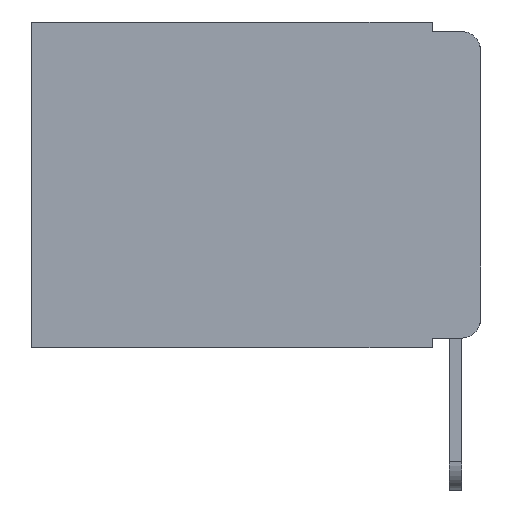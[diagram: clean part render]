
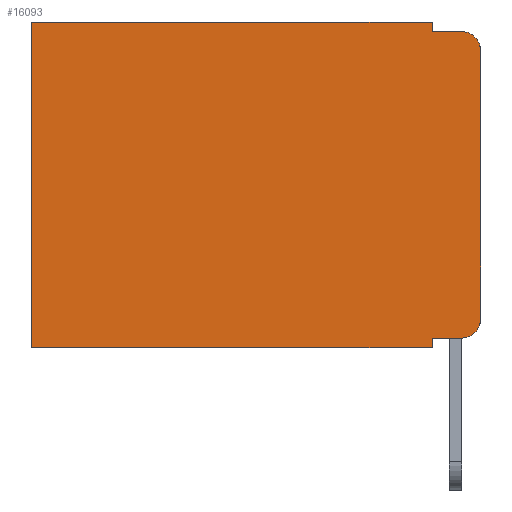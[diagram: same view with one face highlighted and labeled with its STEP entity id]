
A CAD part, left-side view. The second image highlights one B-rep face of the part: STEP entity #16093.
In plain terms, the highlighted planar face has unit normal (-1, 0, 0).
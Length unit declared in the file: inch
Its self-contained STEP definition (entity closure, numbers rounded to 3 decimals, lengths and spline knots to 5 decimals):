
#218 = DIRECTION ( 'NONE',  ( 0., 0., -1. ) ) ;
#620 = DIRECTION ( 'NONE',  ( 0., 0., -1. ) ) ;
#716 = ORIENTED_EDGE ( 'NONE', *, *, #12379, .T. ) ;
#1235 = ORIENTED_EDGE ( 'NONE', *, *, #10543, .T. ) ;
#1444 = VERTEX_POINT ( 'NONE', #15951 ) ;
#1968 = ORIENTED_EDGE ( 'NONE', *, *, #21767, .F. ) ;
#2076 = VECTOR ( 'NONE', #23118, 39.37008 ) ;
#2383 = CARTESIAN_POINT ( 'NONE',  ( 0.298, 0.051, 0. ) ) ;
#2390 = EDGE_CURVE ( 'NONE', #13320, #24098, #7333, .T. ) ;
#2645 = VERTEX_POINT ( 'NONE', #13306 ) ;
#2915 = EDGE_CURVE ( 'NONE', #1444, #13988, #16369, .T. ) ;
#3162 = CARTESIAN_POINT ( 'NONE',  ( 0.298, 0.02, -0.333 ) ) ;
#3163 = LINE ( 'NONE', #13376, #8600 ) ;
#3972 = VERTEX_POINT ( 'NONE', #8825 ) ;
#4665 = ORIENTED_EDGE ( 'NONE', *, *, #17381, .F. ) ;
#4711 = ORIENTED_EDGE ( 'NONE', *, *, #17825, .T. ) ;
#5055 = DIRECTION ( 'NONE',  ( 0., 0., -1. ) ) ;
#5322 = DIRECTION ( 'NONE',  ( 0., 1., 0. ) ) ;
#5402 = VECTOR ( 'NONE', #9149, 39.37008 ) ;
#5779 = EDGE_CURVE ( 'NONE', #12187, #3972, #19331, .T. ) ;
#5966 = ORIENTED_EDGE ( 'NONE', *, *, #2915, .F. ) ;
#6070 = VERTEX_POINT ( 'NONE', #24934 ) ;
#6493 = DIRECTION ( 'NONE',  ( -1., 0., 0. ) ) ;
#6705 = VECTOR ( 'NONE', #22120, 39.37008 ) ;
#7333 = LINE ( 'NONE', #24567, #6705 ) ;
#8185 = LINE ( 'NONE', #17660, #2076 ) ;
#8600 = VECTOR ( 'NONE', #9539, 39.37008 ) ;
#8825 = CARTESIAN_POINT ( 'NONE',  ( 0.298, 0.473, 0. ) ) ;
#8897 = CARTESIAN_POINT ( 'NONE',  ( 0.298, 0.051, 0. ) ) ;
#8924 = PLANE ( 'NONE',  #21454 ) ;
#9149 = DIRECTION ( 'NONE',  ( 0., 0., -1. ) ) ;
#9539 = DIRECTION ( 'NONE',  ( 0., -1., 0. ) ) ;
#10543 = EDGE_CURVE ( 'NONE', #20269, #24098, #13896, .T. ) ;
#10923 = DIRECTION ( 'NONE',  ( 0., 0., -1. ) ) ;
#11085 = DIRECTION ( 'NONE',  ( 0., 0., -1. ) ) ;
#12187 = VERTEX_POINT ( 'NONE', #2383 ) ;
#12370 = DIRECTION ( 'NONE',  ( -1., 0., 0. ) ) ;
#12379 = EDGE_CURVE ( 'NONE', #3972, #2645, #22385, .T. ) ;
#12670 = LINE ( 'NONE', #18305, #21870 ) ;
#13306 = CARTESIAN_POINT ( 'NONE',  ( 0.298, 0.473, -0.343 ) ) ;
#13320 = VERTEX_POINT ( 'NONE', #16192 ) ;
#13339 = FACE_OUTER_BOUND ( 'NONE', #15372, .T. ) ;
#13376 = CARTESIAN_POINT ( 'NONE',  ( 0.298, 0.051, -0.333 ) ) ;
#13896 = CIRCLE ( 'NONE', #24868, 0.02 ) ;
#13988 = VERTEX_POINT ( 'NONE', #21680 ) ;
#14580 = EDGE_CURVE ( 'NONE', #13988, #2645, #8185, .T. ) ;
#14984 = AXIS2_PLACEMENT_3D ( 'NONE', #17973, #6493, #19795 ) ;
#15081 = ORIENTED_EDGE ( 'NONE', *, *, #14580, .F. ) ;
#15102 = CARTESIAN_POINT ( 'NONE',  ( 0.298, 0., 0. ) ) ;
#15372 = EDGE_LOOP ( 'NONE', ( #1968, #1235, #20192, #4665, #15704, #716, #15081, #5966, #17944, #4711 ) ) ;
#15704 = ORIENTED_EDGE ( 'NONE', *, *, #5779, .T. ) ;
#15951 = CARTESIAN_POINT ( 'NONE',  ( 0.298, 0.051, -0.333 ) ) ;
#16093 = ADVANCED_FACE ( 'NONE', ( #13339 ), #8924, .F. ) ;
#16192 = CARTESIAN_POINT ( 'NONE',  ( 0.298, 0.051, -0.01 ) ) ;
#16369 = LINE ( 'NONE', #8897, #5402 ) ;
#16576 = CARTESIAN_POINT ( 'NONE',  ( 0.298, 0., 0. ) ) ;
#17053 = CIRCLE ( 'NONE', #14984, 0.02 ) ;
#17381 = EDGE_CURVE ( 'NONE', #12187, #13320, #12670, .T. ) ;
#17587 = CARTESIAN_POINT ( 'NONE',  ( 0.298, 0., -0.03 ) ) ;
#17660 = CARTESIAN_POINT ( 'NONE',  ( 0.298, 0., -0.343 ) ) ;
#17825 = EDGE_CURVE ( 'NONE', #21234, #6070, #17053, .T. ) ;
#17944 = ORIENTED_EDGE ( 'NONE', *, *, #22685, .T. ) ;
#17973 = CARTESIAN_POINT ( 'NONE',  ( 0.298, 0.02, -0.313 ) ) ;
#18305 = CARTESIAN_POINT ( 'NONE',  ( 0.298, 0.051, 0. ) ) ;
#19294 = VECTOR ( 'NONE', #5055, 39.37008 ) ;
#19331 = LINE ( 'NONE', #15102, #21576 ) ;
#19795 = DIRECTION ( 'NONE',  ( 0., 0., -1. ) ) ;
#20192 = ORIENTED_EDGE ( 'NONE', *, *, #2390, .F. ) ;
#20269 = VERTEX_POINT ( 'NONE', #17587 ) ;
#21234 = VERTEX_POINT ( 'NONE', #3162 ) ;
#21454 = AXIS2_PLACEMENT_3D ( 'NONE', #16576, #22017, #10923 ) ;
#21553 = CARTESIAN_POINT ( 'NONE',  ( 0.298, 0.02, -0.01 ) ) ;
#21576 = VECTOR ( 'NONE', #5322, 39.37008 ) ;
#21680 = CARTESIAN_POINT ( 'NONE',  ( 0.298, 0.051, -0.343 ) ) ;
#21767 = EDGE_CURVE ( 'NONE', #20269, #6070, #24120, .T. ) ;
#21870 = VECTOR ( 'NONE', #620, 39.37008 ) ;
#22017 = DIRECTION ( 'NONE',  ( 1., 0., 0. ) ) ;
#22120 = DIRECTION ( 'NONE',  ( 0., -1., 0. ) ) ;
#22385 = LINE ( 'NONE', #23989, #22960 ) ;
#22685 = EDGE_CURVE ( 'NONE', #1444, #21234, #3163, .T. ) ;
#22960 = VECTOR ( 'NONE', #11085, 39.37008 ) ;
#23118 = DIRECTION ( 'NONE',  ( 0., 1., 0. ) ) ;
#23347 = CARTESIAN_POINT ( 'NONE',  ( 0.298, 0.02, -0.03 ) ) ;
#23927 = CARTESIAN_POINT ( 'NONE',  ( 0.298, 0., 0. ) ) ;
#23989 = CARTESIAN_POINT ( 'NONE',  ( 0.298, 0.473, 0. ) ) ;
#24098 = VERTEX_POINT ( 'NONE', #21553 ) ;
#24120 = LINE ( 'NONE', #23927, #19294 ) ;
#24567 = CARTESIAN_POINT ( 'NONE',  ( 0.298, 0.051, -0.01 ) ) ;
#24868 = AXIS2_PLACEMENT_3D ( 'NONE', #23347, #12370, #218 ) ;
#24934 = CARTESIAN_POINT ( 'NONE',  ( 0.298, 0., -0.313 ) ) ;
